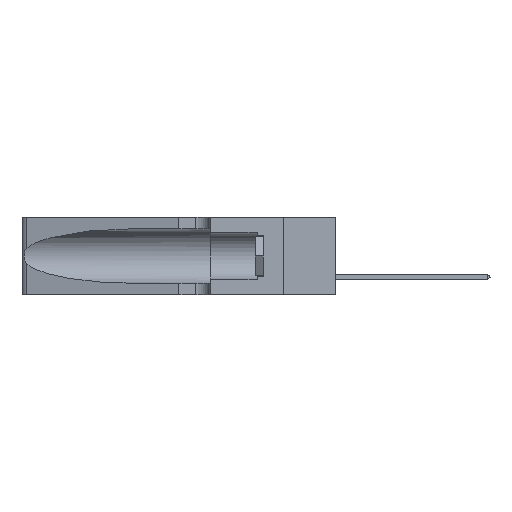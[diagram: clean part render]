
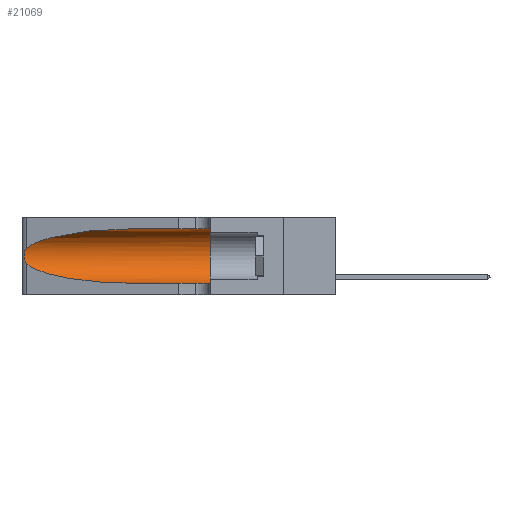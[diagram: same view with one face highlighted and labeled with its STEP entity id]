
A CAD part, left-side view. The second image highlights one B-rep face of the part: STEP entity #21069.
In plain terms, the highlighted cylindrical face has radius 3.308 mm (diameter 6.617 mm), a partial arc.
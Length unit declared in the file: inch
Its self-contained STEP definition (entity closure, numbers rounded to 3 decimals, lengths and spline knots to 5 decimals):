
#770 = ORIENTED_EDGE ( 'NONE', *, *, #31878, .T. ) ;
#1271 = CARTESIAN_POINT ( 'NONE',  ( 0.1305, 0.72297, 0.31525 ) ) ;
#1353 = CARTESIAN_POINT ( 'NONE',  ( 0.25789, 1.23486, 0.15765 ) ) ;
#1675 = CARTESIAN_POINT ( 'NONE',  ( 0.25555, 1.22994, 0.2215 ) ) ;
#3103 =( BOUNDED_CURVE ( )  B_SPLINE_CURVE ( 3, ( #38507, #34839, #17376, #17992 ),
 .UNSPECIFIED., .F., .F. ) 
 B_SPLINE_CURVE_WITH_KNOTS ( ( 4, 4 ),
 ( 3.44316, 4.71239 ),
 .UNSPECIFIED. ) 
 CURVE ( )  GEOMETRIC_REPRESENTATION_ITEM ( )  RATIONAL_B_SPLINE_CURVE ( ( 1., 0.87, 0.87, 1. ) ) 
 REPRESENTATION_ITEM ( '' )  );
#3267 = DIRECTION ( 'NONE',  ( 0., -1., 0. ) ) ;
#3743 = CARTESIAN_POINT ( 'NONE',  ( 0.1305, 0.72297, 0.05475 ) ) ;
#4760 = AXIS2_PLACEMENT_3D ( 'NONE', #8690, #16099, #38447 ) ;
#5046 = CARTESIAN_POINT ( 'NONE',  ( 0.25555, 1.22993, 0.14849 ) ) ;
#6028 = CARTESIAN_POINT ( 'NONE',  ( 0.1305, 0.35, 0.31525 ) ) ;
#6078 = CARTESIAN_POINT ( 'NONE',  ( 0.25487, 1.22718, 0.14631 ) ) ;
#8030 = VERTEX_POINT ( 'NONE', #13213 ) ;
#8680 = CARTESIAN_POINT ( 'NONE',  ( 0.26017, 1.23833, 0.17102 ) ) ;
#8690 = CARTESIAN_POINT ( 'NONE',  ( 0.1305, 0.35, 0.185 ) ) ;
#9525 = CARTESIAN_POINT ( 'NONE',  ( 0.1305, 1.61858, 0.31525 ) ) ;
#11843 = VERTEX_POINT ( 'NONE', #1271 ) ;
#12138 = CARTESIAN_POINT ( 'NONE',  ( 0.26075, 1.23896, 0.178 ) ) ;
#12307 = CARTESIAN_POINT ( 'NONE',  ( 0.25856, 1.23593, 0.16098 ) ) ;
#12463 = CARTESIAN_POINT ( 'NONE',  ( 0.25487, 1.22718, 0.14631 ) ) ;
#12479 = CARTESIAN_POINT ( 'NONE',  ( 0.18966, 0.96281, 0.31525 ) ) ;
#13084 = CARTESIAN_POINT ( 'NONE',  ( 0.2373, 1.15595, 0.28018 ) ) ;
#13213 = CARTESIAN_POINT ( 'NONE',  ( 0.1305, 0.35, 0.05475 ) ) ;
#13694 = VECTOR ( 'NONE', #34908, 39.37008 ) ;
#14093 = EDGE_CURVE ( 'NONE', #11843, #25070, #22849, .T. ) ;
#15935 = CARTESIAN_POINT ( 'NONE',  ( 0.25487, 1.22718, 0.22369 ) ) ;
#16099 = DIRECTION ( 'NONE',  ( 0., 1., 0. ) ) ;
#16464 = ORIENTED_EDGE ( 'NONE', *, *, #38895, .T. ) ;
#17376 = CARTESIAN_POINT ( 'NONE',  ( 0.18966, 0.96281, 0.05475 ) ) ;
#17992 = CARTESIAN_POINT ( 'NONE',  ( 0.1305, 0.72297, 0.05475 ) ) ;
#19603 = CARTESIAN_POINT ( 'NONE',  ( 0.26075, 1.23896, 0.19203 ) ) ;
#19657 = EDGE_CURVE ( 'NONE', #25070, #8030, #31228, .T. ) ;
#19787 = ORIENTED_EDGE ( 'NONE', *, *, #30071, .T. ) ;
#21069 = ADVANCED_FACE ( 'NONE', ( #34576 ), #39670, .F. ) ;
#21133 = EDGE_CURVE ( 'NONE', #35091, #33829, #33465, .T. ) ;
#22849 = LINE ( 'NONE', #9525, #31465 ) ;
#24667 = CARTESIAN_POINT ( 'NONE',  ( 0.1305, 1.61858, 0.05475 ) ) ;
#24799 = CARTESIAN_POINT ( 'NONE',  ( 0.25487, 1.22718, 0.22369 ) ) ;
#25070 = VERTEX_POINT ( 'NONE', #6028 ) ;
#26289 = DIRECTION ( 'NONE',  ( 0., -1., 0. ) ) ;
#27249 = CARTESIAN_POINT ( 'NONE',  ( 0.25487, 1.22718, 0.22369 ) ) ;
#30071 = EDGE_CURVE ( 'NONE', #33829, #36469, #3103, .T. ) ;
#30312 = DIRECTION ( 'NONE',  ( 0., 0., -1. ) ) ;
#30631 = CARTESIAN_POINT ( 'NONE',  ( 0.1305, 0.72297, 0.31525 ) ) ;
#31228 = CIRCLE ( 'NONE', #4760, 0.13025 ) ;
#31465 = VECTOR ( 'NONE', #3267, 39.37008 ) ;
#31878 = EDGE_CURVE ( 'NONE', #11843, #35091, #36393, .T. ) ;
#33465 = B_SPLINE_CURVE_WITH_KNOTS ( 'NONE', 3,
 ( #15935, #1675, #37836, #34162, #37667, #41485, #19603, #12138, #8680, #12307, #1353, #45140, #5046, #12463 ),
 .UNSPECIFIED., .F., .F.,
 ( 4, 2, 2, 2, 2, 2, 4 ),
 ( 0., 0.00027, 0.00053, 0.00107, 0.0016, 0.00187, 0.00214 ),
 .UNSPECIFIED. ) ;
#33829 = VERTEX_POINT ( 'NONE', #6078 ) ;
#33840 = ORIENTED_EDGE ( 'NONE', *, *, #21133, .T. ) ;
#34162 = CARTESIAN_POINT ( 'NONE',  ( 0.25787, 1.23484, 0.2124 ) ) ;
#34576 = FACE_OUTER_BOUND ( 'NONE', #39638, .T. ) ;
#34839 = CARTESIAN_POINT ( 'NONE',  ( 0.2373, 1.15595, 0.08982 ) ) ;
#34908 = DIRECTION ( 'NONE',  ( 0., -1., 0. ) ) ;
#35091 = VERTEX_POINT ( 'NONE', #24799 ) ;
#35549 = AXIS2_PLACEMENT_3D ( 'NONE', #41157, #26289, #30312 ) ;
#36393 =( BOUNDED_CURVE ( )  B_SPLINE_CURVE ( 3, ( #30631, #12479, #13084, #27249 ),
 .UNSPECIFIED., .F., .T. ) 
 B_SPLINE_CURVE_WITH_KNOTS ( ( 4, 4 ),
 ( 1.5708, 2.84003 ),
 .UNSPECIFIED. ) 
 CURVE ( )  GEOMETRIC_REPRESENTATION_ITEM ( )  RATIONAL_B_SPLINE_CURVE ( ( 1., 0.87, 0.87, 1. ) ) 
 REPRESENTATION_ITEM ( '' )  );
#36469 = VERTEX_POINT ( 'NONE', #3743 ) ;
#37667 = CARTESIAN_POINT ( 'NONE',  ( 0.25854, 1.2359, 0.20912 ) ) ;
#37836 = CARTESIAN_POINT ( 'NONE',  ( 0.25639, 1.23184, 0.21858 ) ) ;
#38239 = LINE ( 'NONE', #24667, #13694 ) ;
#38447 = DIRECTION ( 'NONE',  ( 0., 0., 1. ) ) ;
#38507 = CARTESIAN_POINT ( 'NONE',  ( 0.25487, 1.22718, 0.14631 ) ) ;
#38895 = EDGE_CURVE ( 'NONE', #36469, #8030, #38239, .T. ) ;
#39638 = EDGE_LOOP ( 'NONE', ( #770, #33840, #19787, #16464, #40988, #41853 ) ) ;
#39670 = CYLINDRICAL_SURFACE ( 'NONE', #35549, 0.13025 ) ;
#40988 = ORIENTED_EDGE ( 'NONE', *, *, #19657, .F. ) ;
#41157 = CARTESIAN_POINT ( 'NONE',  ( 0.1305, 1.61858, 0.185 ) ) ;
#41485 = CARTESIAN_POINT ( 'NONE',  ( 0.26018, 1.23835, 0.19895 ) ) ;
#41853 = ORIENTED_EDGE ( 'NONE', *, *, #14093, .F. ) ;
#45140 = CARTESIAN_POINT ( 'NONE',  ( 0.25639, 1.23186, 0.15144 ) ) ;
